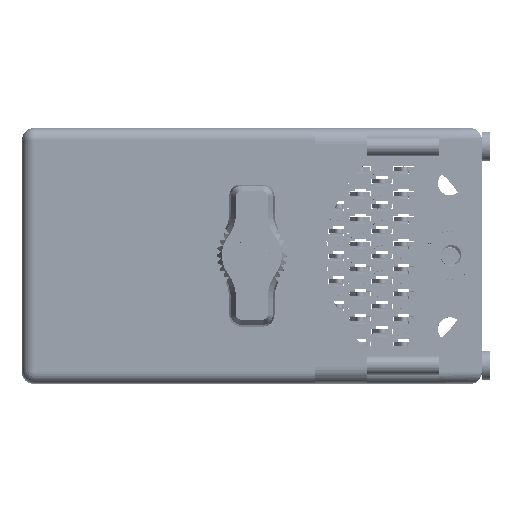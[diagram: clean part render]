
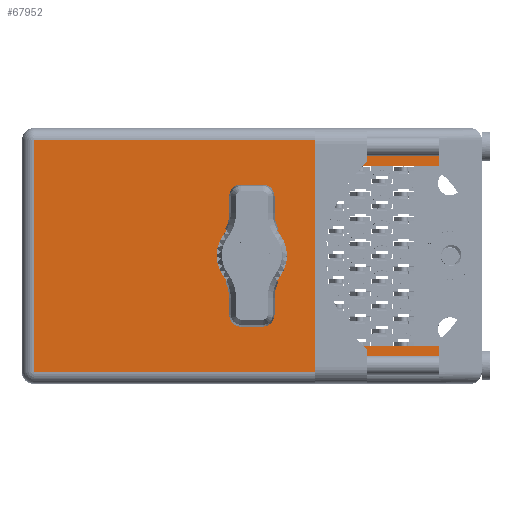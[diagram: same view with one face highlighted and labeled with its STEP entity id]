
A CAD part, top view. The second image highlights one B-rep face of the part: STEP entity #67952.
In plain terms, the highlighted face is planar.
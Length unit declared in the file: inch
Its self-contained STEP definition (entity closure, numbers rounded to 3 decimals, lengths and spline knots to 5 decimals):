
#7 = LINE ( 'NONE', #100506, #97836 ) ;
#4188 = VERTEX_POINT ( 'NONE', #42518 ) ;
#5644 = DIRECTION ( 'NONE',  ( 0., 0., 1. ) ) ;
#8221 = LINE ( 'NONE', #14180, #33406 ) ;
#8348 = VERTEX_POINT ( 'NONE', #25225 ) ;
#8719 = VERTEX_POINT ( 'NONE', #19260 ) ;
#10444 = CARTESIAN_POINT ( 'NONE',  ( 1.1215, 1.93, 0.695 ) ) ;
#11270 = EDGE_CURVE ( 'NONE', #62419, #49678, #92953, .T. ) ;
#11641 = DIRECTION ( 'NONE',  ( 0., 0., 1. ) ) ;
#12934 = VECTOR ( 'NONE', #97989, 39.37008 ) ;
#14180 = CARTESIAN_POINT ( 'NONE',  ( -1.3775, 1.93, -0.695 ) ) ;
#15570 = VERTEX_POINT ( 'NONE', #82981 ) ;
#15735 = CARTESIAN_POINT ( 'NONE',  ( 0., 1.93, 0. ) ) ;
#16242 = ORIENTED_EDGE ( 'NONE', *, *, #101968, .T. ) ;
#17393 = AXIS2_PLACEMENT_3D ( 'NONE', #17700, #61727, #26664 ) ;
#17414 = CARTESIAN_POINT ( 'NONE',  ( 1.1215, 1.93, -0.695 ) ) ;
#17564 = CARTESIAN_POINT ( 'NONE',  ( 1.1215, 1.93, -0.54 ) ) ;
#17700 = CARTESIAN_POINT ( 'NONE',  ( -1.3775, 1.93, -0.765 ) ) ;
#19260 = CARTESIAN_POINT ( 'NONE',  ( 1.1215, 1.93, -0.54 ) ) ;
#21181 = ORIENTED_EDGE ( 'NONE', *, *, #85236, .F. ) ;
#22896 = CARTESIAN_POINT ( 'NONE',  ( 1.1215, 1.93, -0.765 ) ) ;
#23619 = CARTESIAN_POINT ( 'NONE',  ( 0.4075, 1.93, -0.54 ) ) ;
#25210 = CARTESIAN_POINT ( 'NONE',  ( 0.4075, 1.93, 0.54 ) ) ;
#25225 = CARTESIAN_POINT ( 'NONE',  ( 0., 1.93, -0.17 ) ) ;
#25227 = EDGE_LOOP ( 'NONE', ( #57189, #21181 ) ) ;
#26274 = LINE ( 'NONE', #22896, #115671 ) ;
#26664 = DIRECTION ( 'NONE',  ( -1., 0., 0. ) ) ;
#29451 = DIRECTION ( 'NONE',  ( 0., 0., 1. ) ) ;
#30110 = ORIENTED_EDGE ( 'NONE', *, *, #90321, .F. ) ;
#31566 = VERTEX_POINT ( 'NONE', #107250 ) ;
#33406 = VECTOR ( 'NONE', #103197, 39.37008 ) ;
#35260 = EDGE_CURVE ( 'NONE', #75889, #15570, #8221, .T. ) ;
#35705 = VECTOR ( 'NONE', #64189, 39.37008 ) ;
#36192 = ORIENTED_EDGE ( 'NONE', *, *, #42591, .T. ) ;
#37081 = DIRECTION ( 'NONE',  ( 0., 1., 0. ) ) ;
#37492 = CARTESIAN_POINT ( 'NONE',  ( 0., 1.93, 0.17 ) ) ;
#40203 = LINE ( 'NONE', #50142, #45726 ) ;
#42518 = CARTESIAN_POINT ( 'NONE',  ( 1.1215, 1.93, 0.54 ) ) ;
#42591 = EDGE_CURVE ( 'NONE', #31566, #112514, #99111, .T. ) ;
#43160 = AXIS2_PLACEMENT_3D ( 'NONE', #15735, #78135, #60510 ) ;
#43199 = VECTOR ( 'NONE', #65692, 39.37008 ) ;
#43505 = EDGE_CURVE ( 'NONE', #4188, #62419, #40203, .T. ) ;
#45726 = VECTOR ( 'NONE', #76687, 39.37008 ) ;
#48972 = ORIENTED_EDGE ( 'NONE', *, *, #106096, .T. ) ;
#49678 = VERTEX_POINT ( 'NONE', #23619 ) ;
#49942 = VERTEX_POINT ( 'NONE', #37492 ) ;
#50142 = CARTESIAN_POINT ( 'NONE',  ( 1.1215, 1.93, 0.54 ) ) ;
#50810 = DIRECTION ( 'NONE',  ( 0., 0., 1. ) ) ;
#52103 = VECTOR ( 'NONE', #50810, 39.37008 ) ;
#54353 = ORIENTED_EDGE ( 'NONE', *, *, #93062, .F. ) ;
#56823 = CARTESIAN_POINT ( 'NONE',  ( 0.4075, 1.93, -0.54 ) ) ;
#57189 = ORIENTED_EDGE ( 'NONE', *, *, #106136, .F. ) ;
#60087 = CARTESIAN_POINT ( 'NONE',  ( 1.1215, 1.93, -0.765 ) ) ;
#60510 = DIRECTION ( 'NONE',  ( 0., 0., 1. ) ) ;
#61707 = ORIENTED_EDGE ( 'NONE', *, *, #11270, .T. ) ;
#61727 = DIRECTION ( 'NONE',  ( 0., 1., 0. ) ) ;
#62419 = VERTEX_POINT ( 'NONE', #25210 ) ;
#64189 = DIRECTION ( 'NONE',  ( 0., 0., -1. ) ) ;
#65255 = ORIENTED_EDGE ( 'NONE', *, *, #43505, .T. ) ;
#65692 = DIRECTION ( 'NONE',  ( 1., 0., 0. ) ) ;
#67952 = ADVANCED_FACE ( 'NONE', ( #69772, #83854 ), #106358, .T. ) ;
#69772 = FACE_OUTER_BOUND ( 'NONE', #103438, .T. ) ;
#70194 = ORIENTED_EDGE ( 'NONE', *, *, #35260, .T. ) ;
#71803 = CIRCLE ( 'NONE', #43160, 0.17 ) ;
#72744 = AXIS2_PLACEMENT_3D ( 'NONE', #73286, #37081, #11641 ) ;
#73286 = CARTESIAN_POINT ( 'NONE',  ( 0., 1.93, 0. ) ) ;
#75889 = VERTEX_POINT ( 'NONE', #17414 ) ;
#76687 = DIRECTION ( 'NONE',  ( -1., 0., 0. ) ) ;
#78135 = DIRECTION ( 'NONE',  ( 0., 1., 0. ) ) ;
#78593 = LINE ( 'NONE', #17564, #12934 ) ;
#82981 = CARTESIAN_POINT ( 'NONE',  ( -1.3075, 1.93, -0.695 ) ) ;
#83854 = FACE_BOUND ( 'NONE', #25227, .T. ) ;
#85236 = EDGE_CURVE ( 'NONE', #8348, #49942, #71803, .T. ) ;
#85274 = CARTESIAN_POINT ( 'NONE',  ( 1.1215, 1.93, 0.695 ) ) ;
#90321 = EDGE_CURVE ( 'NONE', #4188, #112514, #26274, .T. ) ;
#92953 = LINE ( 'NONE', #56823, #35705 ) ;
#93062 = EDGE_CURVE ( 'NONE', #75889, #8719, #99802, .T. ) ;
#97836 = VECTOR ( 'NONE', #29451, 39.37008 ) ;
#97989 = DIRECTION ( 'NONE',  ( 1., 0., 0. ) ) ;
#99111 = LINE ( 'NONE', #85274, #43199 ) ;
#99802 = LINE ( 'NONE', #60087, #52103 ) ;
#100506 = CARTESIAN_POINT ( 'NONE',  ( -1.3075, 1.93, -0.765 ) ) ;
#101968 = EDGE_CURVE ( 'NONE', #15570, #31566, #7, .T. ) ;
#103197 = DIRECTION ( 'NONE',  ( -1., 0., 0. ) ) ;
#103438 = EDGE_LOOP ( 'NONE', ( #16242, #36192, #30110, #65255, #61707, #48972, #54353, #70194 ) ) ;
#106096 = EDGE_CURVE ( 'NONE', #49678, #8719, #78593, .T. ) ;
#106136 = EDGE_CURVE ( 'NONE', #49942, #8348, #112096, .T. ) ;
#106358 = PLANE ( 'NONE',  #17393 ) ;
#107250 = CARTESIAN_POINT ( 'NONE',  ( -1.3075, 1.93, 0.695 ) ) ;
#112096 = CIRCLE ( 'NONE', #72744, 0.17 ) ;
#112514 = VERTEX_POINT ( 'NONE', #10444 ) ;
#115671 = VECTOR ( 'NONE', #5644, 39.37008 ) ;
